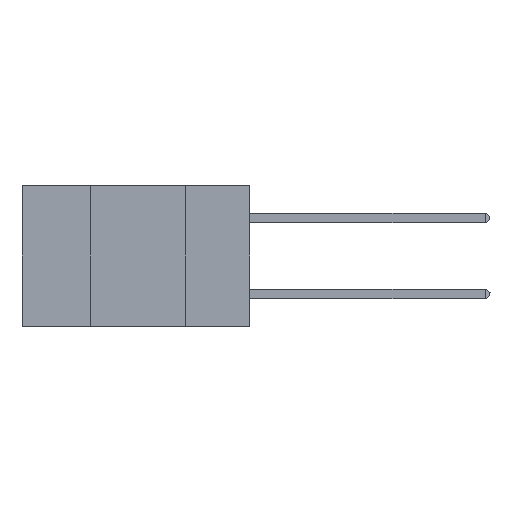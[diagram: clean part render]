
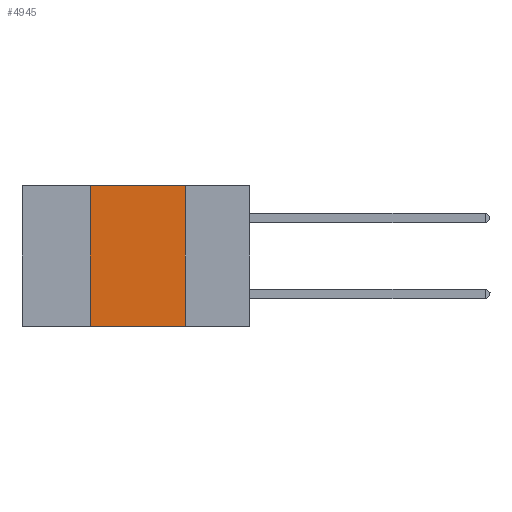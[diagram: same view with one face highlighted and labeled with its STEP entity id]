
A CAD part, left-side view. The second image highlights one B-rep face of the part: STEP entity #4945.
In plain terms, the highlighted planar face has unit normal (-1, 0, 0).
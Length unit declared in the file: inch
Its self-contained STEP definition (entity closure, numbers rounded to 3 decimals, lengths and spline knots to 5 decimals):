
#231 = LINE ( 'NONE', #22473, #19414 ) ;
#752 = EDGE_CURVE ( 'NONE', #9226, #17842, #12384, .T. ) ;
#822 = CARTESIAN_POINT ( 'NONE',  ( 0., 0.42, -0.37 ) ) ;
#1876 = VECTOR ( 'NONE', #23413, 39.37008 ) ;
#2017 = CARTESIAN_POINT ( 'NONE',  ( 0., 0.6, 0. ) ) ;
#4044 = DIRECTION ( 'NONE',  ( 0., -1., 0. ) ) ;
#4945 = ADVANCED_FACE ( 'NONE', ( #7747 ), #11286, .F. ) ;
#5730 = DIRECTION ( 'NONE',  ( 1., 0., 0. ) ) ;
#5810 = DIRECTION ( 'NONE',  ( 0., 0., -1. ) ) ;
#6128 = DIRECTION ( 'NONE',  ( 0., -1., 0. ) ) ;
#7747 = FACE_OUTER_BOUND ( 'NONE', #13568, .T. ) ;
#7799 = ORIENTED_EDGE ( 'NONE', *, *, #7868, .T. ) ;
#7868 = EDGE_CURVE ( 'NONE', #14909, #17842, #231, .T. ) ;
#8651 = ORIENTED_EDGE ( 'NONE', *, *, #752, .F. ) ;
#9226 = VERTEX_POINT ( 'NONE', #10712 ) ;
#9361 = VERTEX_POINT ( 'NONE', #12988 ) ;
#10712 = CARTESIAN_POINT ( 'NONE',  ( 0., 0.17, 0. ) ) ;
#11286 = PLANE ( 'NONE',  #23506 ) ;
#12384 = LINE ( 'NONE', #14356, #1876 ) ;
#12988 = CARTESIAN_POINT ( 'NONE',  ( 0., 0.42, 0. ) ) ;
#13568 = EDGE_LOOP ( 'NONE', ( #8651, #21633, #22336, #7799 ) ) ;
#13619 = EDGE_CURVE ( 'NONE', #14909, #9361, #15000, .T. ) ;
#14109 = LINE ( 'NONE', #21838, #19294 ) ;
#14356 = CARTESIAN_POINT ( 'NONE',  ( 0., 0.17, 0. ) ) ;
#14420 = EDGE_CURVE ( 'NONE', #9361, #9226, #14109, .T. ) ;
#14909 = VERTEX_POINT ( 'NONE', #822 ) ;
#15000 = LINE ( 'NONE', #19638, #23673 ) ;
#15516 = CARTESIAN_POINT ( 'NONE',  ( 0., 0.17, -0.37 ) ) ;
#15851 = DIRECTION ( 'NONE',  ( 0., 0., 1. ) ) ;
#17842 = VERTEX_POINT ( 'NONE', #15516 ) ;
#19294 = VECTOR ( 'NONE', #4044, 39.37008 ) ;
#19414 = VECTOR ( 'NONE', #6128, 39.37008 ) ;
#19638 = CARTESIAN_POINT ( 'NONE',  ( 0., 0.42, 0. ) ) ;
#21633 = ORIENTED_EDGE ( 'NONE', *, *, #14420, .F. ) ;
#21838 = CARTESIAN_POINT ( 'NONE',  ( 0., 0.6, 0. ) ) ;
#22336 = ORIENTED_EDGE ( 'NONE', *, *, #13619, .F. ) ;
#22473 = CARTESIAN_POINT ( 'NONE',  ( 0., 0.6, -0.37 ) ) ;
#23413 = DIRECTION ( 'NONE',  ( 0., 0., -1. ) ) ;
#23506 = AXIS2_PLACEMENT_3D ( 'NONE', #2017, #5730, #5810 ) ;
#23673 = VECTOR ( 'NONE', #15851, 39.37008 ) ;
